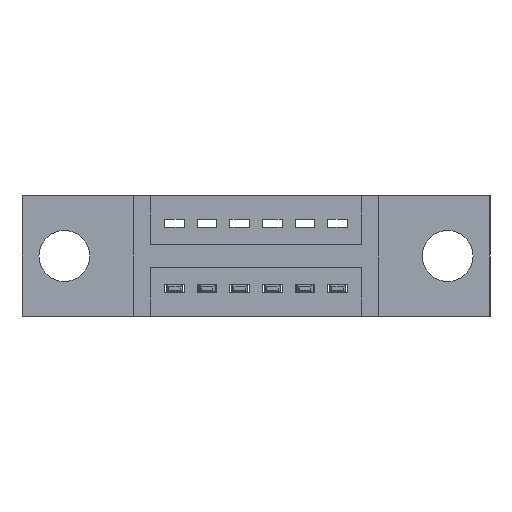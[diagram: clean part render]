
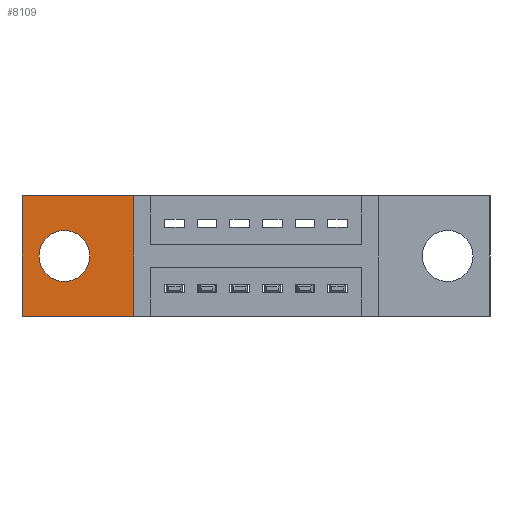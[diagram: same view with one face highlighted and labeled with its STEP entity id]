
A CAD part, front view. The second image highlights one B-rep face of the part: STEP entity #8109.
In plain terms, the highlighted planar face has unit normal (0, -1, 0).
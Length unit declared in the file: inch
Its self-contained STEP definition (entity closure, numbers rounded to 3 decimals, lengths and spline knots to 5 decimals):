
#143 = EDGE_CURVE ( 'NONE', #5224, #1161, #4453, .T. ) ;
#193 = VERTEX_POINT ( 'NONE', #4205 ) ;
#259 = FACE_OUTER_BOUND ( 'NONE', #2725, .T. ) ;
#343 = LINE ( 'NONE', #1771, #5887 ) ;
#379 = FACE_BOUND ( 'NONE', #4904, .T. ) ;
#598 = CARTESIAN_POINT ( 'NONE',  ( 0.13, 0.11, -0.185 ) ) ;
#723 = ORIENTED_EDGE ( 'NONE', *, *, #143, .F. ) ;
#766 = VERTEX_POINT ( 'NONE', #9274 ) ;
#931 = EDGE_CURVE ( 'NONE', #1161, #5224, #4661, .T. ) ;
#1044 = ORIENTED_EDGE ( 'NONE', *, *, #2765, .T. ) ;
#1154 = CARTESIAN_POINT ( 'NONE',  ( 0.13, 0.11, -0.107 ) ) ;
#1161 = VERTEX_POINT ( 'NONE', #1154 ) ;
#1182 = LINE ( 'NONE', #6497, #4388 ) ;
#1188 = AXIS2_PLACEMENT_3D ( 'NONE', #7999, #4397, #7899 ) ;
#1311 = VERTEX_POINT ( 'NONE', #6322 ) ;
#1771 = CARTESIAN_POINT ( 'NONE',  ( 0., 0.11, 0. ) ) ;
#2034 = DIRECTION ( 'NONE',  ( 0., 0., 1. ) ) ;
#2105 = DIRECTION ( 'NONE',  ( 0., 0., -1. ) ) ;
#2200 = CARTESIAN_POINT ( 'NONE',  ( 0., 0.11, -0.37 ) ) ;
#2234 = DIRECTION ( 'NONE',  ( -1., 0., 0. ) ) ;
#2725 = EDGE_LOOP ( 'NONE', ( #1044, #8122, #7599, #4772 ) ) ;
#2765 = EDGE_CURVE ( 'NONE', #1311, #5869, #7749, .T. ) ;
#3006 = EDGE_CURVE ( 'NONE', #193, #766, #1182, .T. ) ;
#3531 = ORIENTED_EDGE ( 'NONE', *, *, #931, .F. ) ;
#3643 = LINE ( 'NONE', #2200, #4231 ) ;
#3912 = VECTOR ( 'NONE', #6882, 39.37008 ) ;
#4205 = CARTESIAN_POINT ( 'NONE',  ( 0.3425, 0.11, -0.37 ) ) ;
#4231 = VECTOR ( 'NONE', #4523, 39.37008 ) ;
#4243 = DIRECTION ( 'NONE',  ( 0., -1., 0. ) ) ;
#4388 = VECTOR ( 'NONE', #2034, 39.37008 ) ;
#4397 = DIRECTION ( 'NONE',  ( 0., -1., 0. ) ) ;
#4453 = CIRCLE ( 'NONE', #7071, 0.078 ) ;
#4523 = DIRECTION ( 'NONE',  ( 1., 0., 0. ) ) ;
#4661 = CIRCLE ( 'NONE', #1188, 0.078 ) ;
#4772 = ORIENTED_EDGE ( 'NONE', *, *, #5111, .T. ) ;
#4904 = EDGE_LOOP ( 'NONE', ( #3531, #723 ) ) ;
#5111 = EDGE_CURVE ( 'NONE', #766, #1311, #343, .T. ) ;
#5224 = VERTEX_POINT ( 'NONE', #9277 ) ;
#5400 = CARTESIAN_POINT ( 'NONE',  ( 0., 0.11, 0. ) ) ;
#5683 = PLANE ( 'NONE',  #6085 ) ;
#5869 = VERTEX_POINT ( 'NONE', #9160 ) ;
#5887 = VECTOR ( 'NONE', #2234, 39.37008 ) ;
#6085 = AXIS2_PLACEMENT_3D ( 'NONE', #6505, #7215, #2105 ) ;
#6322 = CARTESIAN_POINT ( 'NONE',  ( 0., 0.11, 0. ) ) ;
#6497 = CARTESIAN_POINT ( 'NONE',  ( 0.3425, 0.11, 0. ) ) ;
#6505 = CARTESIAN_POINT ( 'NONE',  ( 0., 0.11, -0.37 ) ) ;
#6882 = DIRECTION ( 'NONE',  ( 0., 0., -1. ) ) ;
#7071 = AXIS2_PLACEMENT_3D ( 'NONE', #598, #4243, #7727 ) ;
#7215 = DIRECTION ( 'NONE',  ( 0., -1., 0. ) ) ;
#7599 = ORIENTED_EDGE ( 'NONE', *, *, #3006, .T. ) ;
#7727 = DIRECTION ( 'NONE',  ( 0., 0., -1. ) ) ;
#7749 = LINE ( 'NONE', #5400, #3912 ) ;
#7899 = DIRECTION ( 'NONE',  ( 0., 0., -1. ) ) ;
#7999 = CARTESIAN_POINT ( 'NONE',  ( 0.13, 0.11, -0.185 ) ) ;
#8109 = ADVANCED_FACE ( 'NONE', ( #379, #259 ), #5683, .T. ) ;
#8122 = ORIENTED_EDGE ( 'NONE', *, *, #8222, .T. ) ;
#8222 = EDGE_CURVE ( 'NONE', #5869, #193, #3643, .T. ) ;
#9160 = CARTESIAN_POINT ( 'NONE',  ( 0., 0.11, -0.37 ) ) ;
#9274 = CARTESIAN_POINT ( 'NONE',  ( 0.3425, 0.11, 0. ) ) ;
#9277 = CARTESIAN_POINT ( 'NONE',  ( 0.13, 0.11, -0.263 ) ) ;
